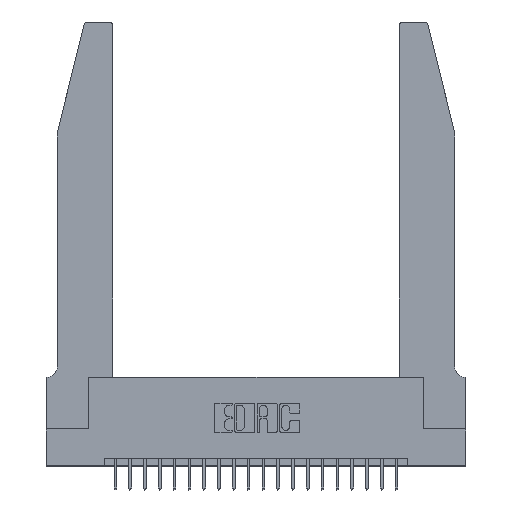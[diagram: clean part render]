
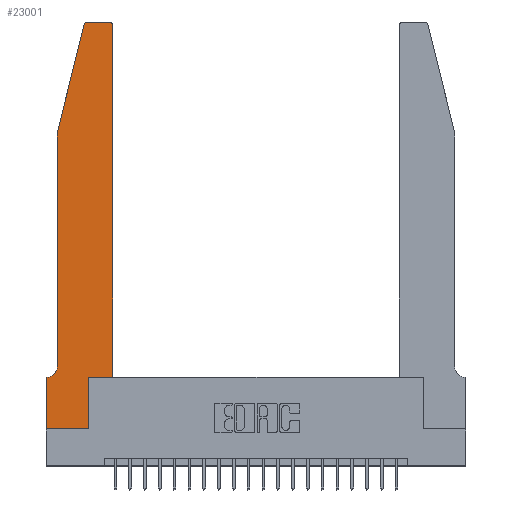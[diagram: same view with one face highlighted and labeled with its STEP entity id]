
A CAD part, top view. The second image highlights one B-rep face of the part: STEP entity #23001.
In plain terms, the highlighted planar face has unit normal (0, 0, 1).
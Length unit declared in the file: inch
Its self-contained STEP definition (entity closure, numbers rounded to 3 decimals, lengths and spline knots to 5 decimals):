
#12 = VERTEX_POINT ( 'NONE', #8131 ) ;
#128 = LINE ( 'NONE', #16207, #12294 ) ;
#191 = CARTESIAN_POINT ( 'NONE',  ( 0.0755, 0.42, 0.37 ) ) ;
#510 = VECTOR ( 'NONE', #2492, 39.37008 ) ;
#861 = DIRECTION ( 'NONE',  ( 1., 0., 0. ) ) ;
#1151 = ORIENTED_EDGE ( 'NONE', *, *, #9173, .T. ) ;
#1391 = CARTESIAN_POINT ( 'NONE',  ( 0.2865, 0., 0.37 ) ) ;
#1610 = ORIENTED_EDGE ( 'NONE', *, *, #11060, .T. ) ;
#1796 = VECTOR ( 'NONE', #22215, 39.37008 ) ;
#1907 = CARTESIAN_POINT ( 'NONE',  ( 0.4205, 2.72, 0.37 ) ) ;
#2202 = LINE ( 'NONE', #11505, #17242 ) ;
#2216 = VERTEX_POINT ( 'NONE', #2315 ) ;
#2315 = CARTESIAN_POINT ( 'NONE',  ( 0.4205, 2.75, 0.37 ) ) ;
#2492 = DIRECTION ( 'NONE',  ( 1., 0., 0. ) ) ;
#2495 = VERTEX_POINT ( 'NONE', #191 ) ;
#3441 = CARTESIAN_POINT ( 'NONE',  ( 0.2865, 0.35, 0.37 ) ) ;
#3810 = VERTEX_POINT ( 'NONE', #19811 ) ;
#4579 = ORIENTED_EDGE ( 'NONE', *, *, #23488, .T. ) ;
#4701 = ORIENTED_EDGE ( 'NONE', *, *, #9334, .T. ) ;
#4974 = DIRECTION ( 'NONE',  ( -1., 0., 0. ) ) ;
#5354 = LINE ( 'NONE', #22596, #510 ) ;
#5412 = VERTEX_POINT ( 'NONE', #7053 ) ;
#5896 = DIRECTION ( 'NONE',  ( -1., 0., 0. ) ) ;
#6035 = EDGE_CURVE ( 'NONE', #14896, #2495, #2202, .T. ) ;
#6129 = ORIENTED_EDGE ( 'NONE', *, *, #14850, .T. ) ;
#6256 = PLANE ( 'NONE',  #19478 ) ;
#6384 = DIRECTION ( 'NONE',  ( 0., -1., 0. ) ) ;
#6603 = LINE ( 'NONE', #13452, #1796 ) ;
#6788 = DIRECTION ( 'NONE',  ( -0.239, -0.971, 0. ) ) ;
#7053 = CARTESIAN_POINT ( 'NONE',  ( 0., 0.35, 0.37 ) ) ;
#7148 = AXIS2_PLACEMENT_3D ( 'NONE', #16762, #18444, #22035 ) ;
#7219 = ORIENTED_EDGE ( 'NONE', *, *, #12145, .T. ) ;
#7232 = CARTESIAN_POINT ( 'NONE',  ( 0.0055, 0.35, 0.37 ) ) ;
#7784 = VECTOR ( 'NONE', #20363, 39.37008 ) ;
#7950 = CARTESIAN_POINT ( 'NONE',  ( 0.0055, 0.42, 0.37 ) ) ;
#8131 = CARTESIAN_POINT ( 'NONE',  ( 0.4505, 2.72, 0.37 ) ) ;
#9076 = DIRECTION ( 'NONE',  ( 0., -1., 0. ) ) ;
#9173 = EDGE_CURVE ( 'NONE', #2495, #14329, #13409, .T. ) ;
#9177 = ORIENTED_EDGE ( 'NONE', *, *, #22853, .T. ) ;
#9334 = EDGE_CURVE ( 'NONE', #18705, #3810, #11106, .T. ) ;
#9335 = CARTESIAN_POINT ( 'NONE',  ( 0.4505, 0.35, 0.37 ) ) ;
#9736 = CARTESIAN_POINT ( 'NONE',  ( 0., 0.35, 0.37 ) ) ;
#9883 = ORIENTED_EDGE ( 'NONE', *, *, #21237, .T. ) ;
#10207 = LINE ( 'NONE', #16498, #10768 ) ;
#10214 = VERTEX_POINT ( 'NONE', #12472 ) ;
#10702 = DIRECTION ( 'NONE',  ( 0., 0., 1. ) ) ;
#10768 = VECTOR ( 'NONE', #22162, 39.37008 ) ;
#11060 = EDGE_CURVE ( 'NONE', #14206, #18705, #5354, .T. ) ;
#11106 = LINE ( 'NONE', #3441, #20222 ) ;
#11305 = ORIENTED_EDGE ( 'NONE', *, *, #17663, .T. ) ;
#11489 = VERTEX_POINT ( 'NONE', #22043 ) ;
#11505 = CARTESIAN_POINT ( 'NONE',  ( 0.0755, 2., 0.37 ) ) ;
#11538 = DIRECTION ( 'NONE',  ( 0., 0., 1. ) ) ;
#11558 = CARTESIAN_POINT ( 'NONE',  ( 0.2605, 2.75, 0.37 ) ) ;
#11886 = CARTESIAN_POINT ( 'NONE',  ( 0.284, 2.75, 0.37 ) ) ;
#12099 = VECTOR ( 'NONE', #5896, 39.37008 ) ;
#12145 = EDGE_CURVE ( 'NONE', #18618, #10214, #21470, .T. ) ;
#12294 = VECTOR ( 'NONE', #9076, 39.37008 ) ;
#12472 = CARTESIAN_POINT ( 'NONE',  ( 0.25487, 2.72718, 0.37 ) ) ;
#12549 = AXIS2_PLACEMENT_3D ( 'NONE', #7950, #13826, #4974 ) ;
#13319 = ORIENTED_EDGE ( 'NONE', *, *, #6035, .T. ) ;
#13409 = CIRCLE ( 'NONE', #12549, 0.07 ) ;
#13452 = CARTESIAN_POINT ( 'NONE',  ( 0.0755, 0.35, 0.37 ) ) ;
#13802 = CARTESIAN_POINT ( 'NONE',  ( 0., 0., 0.37 ) ) ;
#13826 = DIRECTION ( 'NONE',  ( 0., 0., -1. ) ) ;
#14206 = VERTEX_POINT ( 'NONE', #13802 ) ;
#14329 = VERTEX_POINT ( 'NONE', #7232 ) ;
#14381 = LINE ( 'NONE', #11558, #12099 ) ;
#14850 = EDGE_CURVE ( 'NONE', #10214, #14896, #17376, .T. ) ;
#14896 = VERTEX_POINT ( 'NONE', #23229 ) ;
#15111 = FACE_OUTER_BOUND ( 'NONE', #21134, .T. ) ;
#15354 = AXIS2_PLACEMENT_3D ( 'NONE', #1907, #10702, #18159 ) ;
#16207 = CARTESIAN_POINT ( 'NONE',  ( 0., 0., 0.37 ) ) ;
#16498 = CARTESIAN_POINT ( 'NONE',  ( 0.4505, 0.35, 0.37 ) ) ;
#16762 = CARTESIAN_POINT ( 'NONE',  ( 0.284, 2.72, 0.37 ) ) ;
#17242 = VECTOR ( 'NONE', #6384, 39.37008 ) ;
#17376 = LINE ( 'NONE', #17662, #22234 ) ;
#17662 = CARTESIAN_POINT ( 'NONE',  ( 0.0755, 2., 0.37 ) ) ;
#17663 = EDGE_CURVE ( 'NONE', #14329, #5412, #6603, .T. ) ;
#18159 = DIRECTION ( 'NONE',  ( 1., 0., 0. ) ) ;
#18444 = DIRECTION ( 'NONE',  ( 0., 0., 1. ) ) ;
#18598 = ORIENTED_EDGE ( 'NONE', *, *, #18986, .T. ) ;
#18618 = VERTEX_POINT ( 'NONE', #11886 ) ;
#18705 = VERTEX_POINT ( 'NONE', #1391 ) ;
#18986 = EDGE_CURVE ( 'NONE', #11489, #12, #10207, .T. ) ;
#19478 = AXIS2_PLACEMENT_3D ( 'NONE', #9736, #11538, #861 ) ;
#19811 = CARTESIAN_POINT ( 'NONE',  ( 0.2865, 0.35, 0.37 ) ) ;
#19997 = LINE ( 'NONE', #9335, #7784 ) ;
#20222 = VECTOR ( 'NONE', #21586, 39.37008 ) ;
#20363 = DIRECTION ( 'NONE',  ( 1., 0., 0. ) ) ;
#20945 = ORIENTED_EDGE ( 'NONE', *, *, #22629, .T. ) ;
#21134 = EDGE_LOOP ( 'NONE', ( #9883, #7219, #6129, #13319, #1151, #11305, #4579, #1610, #4701, #9177, #18598, #20945 ) ) ;
#21237 = EDGE_CURVE ( 'NONE', #2216, #18618, #14381, .T. ) ;
#21470 = CIRCLE ( 'NONE', #7148, 0.03 ) ;
#21586 = DIRECTION ( 'NONE',  ( 0., 1., 0. ) ) ;
#22035 = DIRECTION ( 'NONE',  ( 1., 0., 0. ) ) ;
#22043 = CARTESIAN_POINT ( 'NONE',  ( 0.4505, 0.35, 0.37 ) ) ;
#22162 = DIRECTION ( 'NONE',  ( 0., 1., 0. ) ) ;
#22215 = DIRECTION ( 'NONE',  ( -1., 0., 0. ) ) ;
#22234 = VECTOR ( 'NONE', #6788, 39.37008 ) ;
#22297 = CIRCLE ( 'NONE', #15354, 0.03 ) ;
#22596 = CARTESIAN_POINT ( 'NONE',  ( 0., 0., 0.37 ) ) ;
#22629 = EDGE_CURVE ( 'NONE', #12, #2216, #22297, .T. ) ;
#22853 = EDGE_CURVE ( 'NONE', #3810, #11489, #19997, .T. ) ;
#23001 = ADVANCED_FACE ( 'NONE', ( #15111 ), #6256, .T. ) ;
#23229 = CARTESIAN_POINT ( 'NONE',  ( 0.0755, 2., 0.37 ) ) ;
#23488 = EDGE_CURVE ( 'NONE', #5412, #14206, #128, .T. ) ;
